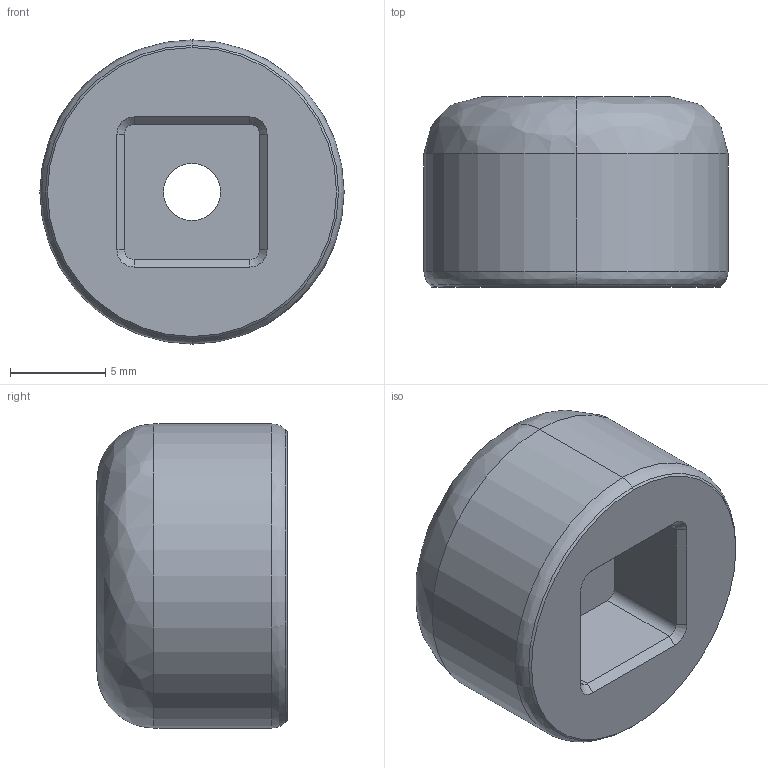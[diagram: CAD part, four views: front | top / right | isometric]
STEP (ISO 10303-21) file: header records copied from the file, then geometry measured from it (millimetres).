
FILE_DESCRIPTION (( 'STEP AP203' ), '1' );
FILE_NAME ('BUTTON.STEP', '2020-09-28T01:15:34', ( '' ), ( '' ), 'SwSTEP 2.0', 'SolidWorks 2019', '' );
FILE_SCHEMA (( 'CONFIG_CONTROL_DESIGN' ));
Length unit declared in the file: millimetre
Products named in the file (1): BUTTON
Bounding box: 16 x 10 x 16 mm (x, y, z)
Volume: 1628.1 mm3; surface area: 986.3 mm2
Topology: 1 solids, 1 shells, 29 faces, 64 edges, 38 vertices
Faces by surface type: plane 11, cylinder 8, cone 6, bspline 4
Entity records: 914 total; most frequent: CARTESIAN_POINT 203, DIRECTION 137, ORIENTED_EDGE 128, EDGE_CURVE 64, AXIS2_PLACEMENT_3D 54, VERTEX_POINT 38, EDGE_LOOP 32, FACE_OUTER_BOUND 29
